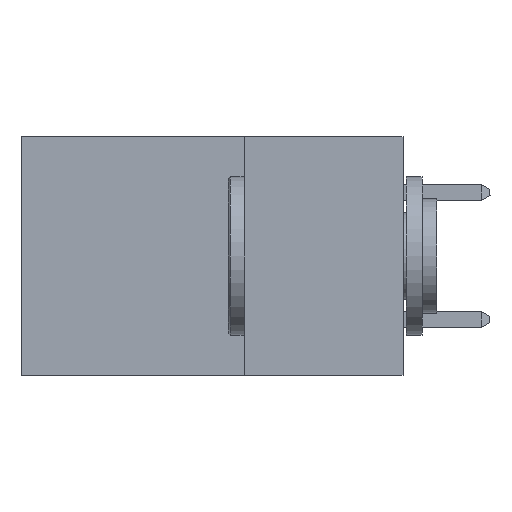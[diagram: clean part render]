
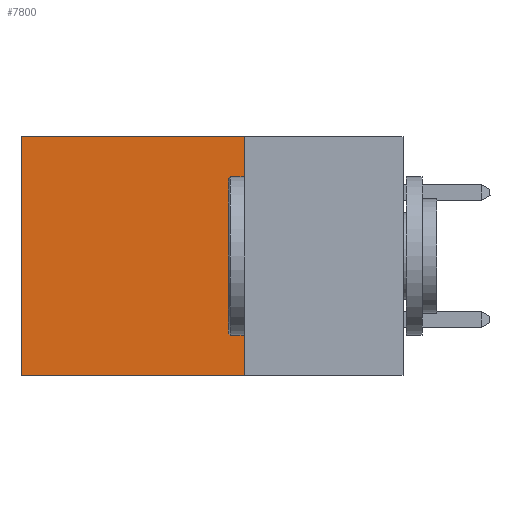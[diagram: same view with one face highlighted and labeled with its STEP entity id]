
A CAD part, left-side view. The second image highlights one B-rep face of the part: STEP entity #7800.
In plain terms, the highlighted planar face has unit normal (-1, 0, 0).
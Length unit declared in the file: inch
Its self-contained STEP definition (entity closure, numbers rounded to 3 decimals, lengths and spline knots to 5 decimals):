
#121 = ORIENTED_EDGE ( 'NONE', *, *, #460, .F. ) ;
#142 = AXIS2_PLACEMENT_3D ( 'NONE', #7641, #7585, #6260 ) ;
#460 = EDGE_CURVE ( 'NONE', #759, #2035, #7332, .T. ) ;
#759 = VERTEX_POINT ( 'NONE', #1217 ) ;
#834 = CARTESIAN_POINT ( 'NONE',  ( 0.2875, 0.25, -0.375 ) ) ;
#1026 = VECTOR ( 'NONE', #2215, 39.37008 ) ;
#1217 = CARTESIAN_POINT ( 'NONE',  ( 0.2875, 0.25, 0. ) ) ;
#1263 = LINE ( 'NONE', #6270, #7132 ) ;
#1340 = CARTESIAN_POINT ( 'NONE',  ( 0.2875, 0.25, -0.375 ) ) ;
#1483 = EDGE_LOOP ( 'NONE', ( #8115, #6242, #121, #2411 ) ) ;
#1566 = DIRECTION ( 'NONE',  ( 0., 1., 0. ) ) ;
#2035 = VERTEX_POINT ( 'NONE', #1340 ) ;
#2215 = DIRECTION ( 'NONE',  ( 0., 1., 0. ) ) ;
#2411 = ORIENTED_EDGE ( 'NONE', *, *, #7313, .T. ) ;
#2493 = DIRECTION ( 'NONE',  ( 0., 0., -1. ) ) ;
#2690 = PLANE ( 'NONE',  #142 ) ;
#2898 = CARTESIAN_POINT ( 'NONE',  ( 0.2875, 0.6, -0.375 ) ) ;
#3606 = VERTEX_POINT ( 'NONE', #5719 ) ;
#4014 = VECTOR ( 'NONE', #2493, 39.37008 ) ;
#4226 = VECTOR ( 'NONE', #5703, 39.37008 ) ;
#4350 = CARTESIAN_POINT ( 'NONE',  ( 0.2875, 0.25, -0.375 ) ) ;
#4683 = FACE_OUTER_BOUND ( 'NONE', #1483, .T. ) ;
#5703 = DIRECTION ( 'NONE',  ( 0., 0., -1. ) ) ;
#5719 = CARTESIAN_POINT ( 'NONE',  ( 0.2875, 0.6, 0. ) ) ;
#6242 = ORIENTED_EDGE ( 'NONE', *, *, #7345, .F. ) ;
#6247 = LINE ( 'NONE', #4350, #1026 ) ;
#6260 = DIRECTION ( 'NONE',  ( 0., 0., -1. ) ) ;
#6270 = CARTESIAN_POINT ( 'NONE',  ( 0.2875, 0.25, 0. ) ) ;
#7055 = CARTESIAN_POINT ( 'NONE',  ( 0.2875, 0.6, -0.375 ) ) ;
#7105 = LINE ( 'NONE', #7055, #4226 ) ;
#7132 = VECTOR ( 'NONE', #1566, 39.37008 ) ;
#7313 = EDGE_CURVE ( 'NONE', #759, #3606, #1263, .T. ) ;
#7332 = LINE ( 'NONE', #834, #4014 ) ;
#7345 = EDGE_CURVE ( 'NONE', #2035, #7375, #6247, .T. ) ;
#7375 = VERTEX_POINT ( 'NONE', #2898 ) ;
#7585 = DIRECTION ( 'NONE',  ( 1., 0., 0. ) ) ;
#7641 = CARTESIAN_POINT ( 'NONE',  ( 0.2875, 0.25, -0.375 ) ) ;
#7800 = ADVANCED_FACE ( 'NONE', ( #4683 ), #2690, .F. ) ;
#8115 = ORIENTED_EDGE ( 'NONE', *, *, #8446, .T. ) ;
#8446 = EDGE_CURVE ( 'NONE', #3606, #7375, #7105, .T. ) ;
